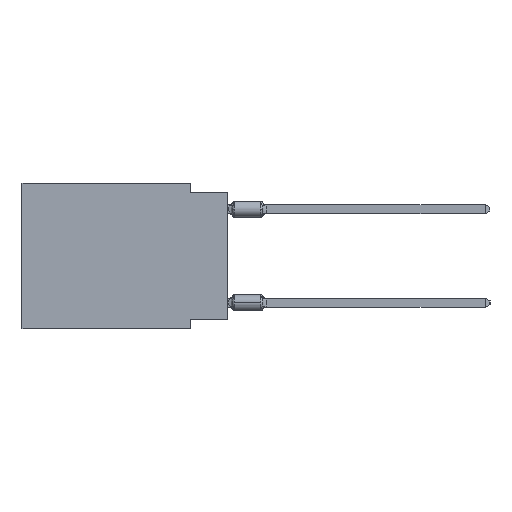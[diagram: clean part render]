
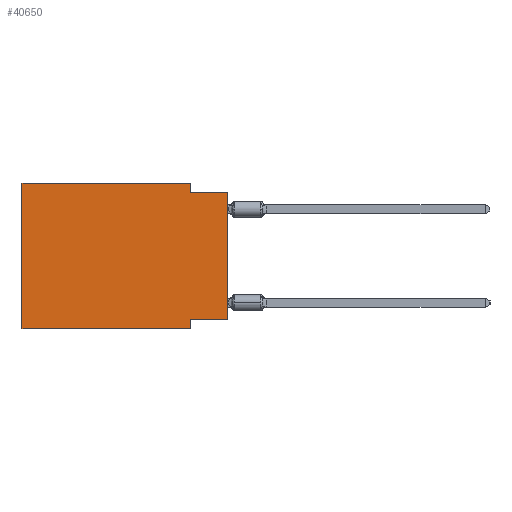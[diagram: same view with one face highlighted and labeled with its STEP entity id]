
A CAD part, left-side view. The second image highlights one B-rep face of the part: STEP entity #40650.
In plain terms, the highlighted planar face has unit normal (-1, 0, 0).
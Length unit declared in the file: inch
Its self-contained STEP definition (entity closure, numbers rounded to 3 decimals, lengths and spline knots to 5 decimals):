
#1346 = VERTEX_POINT ( 'NONE', #27940 ) ;
#1482 = VERTEX_POINT ( 'NONE', #6366 ) ;
#2397 = CARTESIAN_POINT ( 'NONE',  ( 0., 0., -0.025 ) ) ;
#2443 = CARTESIAN_POINT ( 'NONE',  ( 0., 0.1, -0.025 ) ) ;
#3744 = LINE ( 'NONE', #27903, #15398 ) ;
#4629 = FACE_OUTER_BOUND ( 'NONE', #20143, .T. ) ;
#5281 = EDGE_CURVE ( 'NONE', #19329, #8664, #17455, .T. ) ;
#5572 = LINE ( 'NONE', #14890, #19113 ) ;
#6366 = CARTESIAN_POINT ( 'NONE',  ( 0., 0.55, 0. ) ) ;
#7460 = EDGE_CURVE ( 'NONE', #8079, #25161, #27578, .T. ) ;
#7664 = CARTESIAN_POINT ( 'NONE',  ( 0., 0.1, 0. ) ) ;
#8079 = VERTEX_POINT ( 'NONE', #2443 ) ;
#8664 = VERTEX_POINT ( 'NONE', #26353 ) ;
#9581 = CARTESIAN_POINT ( 'NONE',  ( 0., 0., 0. ) ) ;
#10583 = DIRECTION ( 'NONE',  ( 0., 1., 0. ) ) ;
#11356 = EDGE_CURVE ( 'NONE', #19803, #8079, #24972, .T. ) ;
#11784 = VECTOR ( 'NONE', #38459, 39.37008 ) ;
#13032 = ORIENTED_EDGE ( 'NONE', *, *, #17229, .F. ) ;
#13084 = ORIENTED_EDGE ( 'NONE', *, *, #11356, .F. ) ;
#13120 = DIRECTION ( 'NONE',  ( 0., 0., 1. ) ) ;
#14030 = ORIENTED_EDGE ( 'NONE', *, *, #5281, .F. ) ;
#14487 = CARTESIAN_POINT ( 'NONE',  ( 0., 0.55, 0. ) ) ;
#14691 = ORIENTED_EDGE ( 'NONE', *, *, #30767, .T. ) ;
#14890 = CARTESIAN_POINT ( 'NONE',  ( 0., 0.55, 0. ) ) ;
#15280 = EDGE_CURVE ( 'NONE', #20701, #1482, #5572, .T. ) ;
#15398 = VECTOR ( 'NONE', #38090, 39.37008 ) ;
#17229 = EDGE_CURVE ( 'NONE', #1482, #19803, #20938, .T. ) ;
#17455 = LINE ( 'NONE', #24131, #42381 ) ;
#17495 = PLANE ( 'NONE',  #17499 ) ;
#17498 = LINE ( 'NONE', #31476, #43654 ) ;
#17499 = AXIS2_PLACEMENT_3D ( 'NONE', #18152, #21281, #35247 ) ;
#18152 = CARTESIAN_POINT ( 'NONE',  ( 0., 0.55, 0. ) ) ;
#19113 = VECTOR ( 'NONE', #41721, 39.37008 ) ;
#19329 = VERTEX_POINT ( 'NONE', #29270 ) ;
#19803 = VERTEX_POINT ( 'NONE', #32311 ) ;
#20143 = EDGE_LOOP ( 'NONE', ( #14691, #35394, #13084, #13032, #29290, #38434, #33197, #14030 ) ) ;
#20701 = VERTEX_POINT ( 'NONE', #28486 ) ;
#20938 = LINE ( 'NONE', #14487, #11784 ) ;
#21281 = DIRECTION ( 'NONE',  ( 1., 0., 0. ) ) ;
#21282 = DIRECTION ( 'NONE',  ( 0., -1., 0. ) ) ;
#23919 = EDGE_CURVE ( 'NONE', #20701, #1346, #17498, .T. ) ;
#24131 = CARTESIAN_POINT ( 'NONE',  ( 0., 0., -0.365 ) ) ;
#24916 = EDGE_CURVE ( 'NONE', #8664, #1346, #3744, .T. ) ;
#24972 = LINE ( 'NONE', #7664, #25889 ) ;
#25161 = VERTEX_POINT ( 'NONE', #2397 ) ;
#25889 = VECTOR ( 'NONE', #28741, 39.37008 ) ;
#26353 = CARTESIAN_POINT ( 'NONE',  ( 0., 0.1, -0.365 ) ) ;
#27141 = DIRECTION ( 'NONE',  ( 0., -1., 0. ) ) ;
#27578 = LINE ( 'NONE', #40445, #36889 ) ;
#27903 = CARTESIAN_POINT ( 'NONE',  ( 0., 0.1, -0.39 ) ) ;
#27940 = CARTESIAN_POINT ( 'NONE',  ( 0., 0.1, -0.39 ) ) ;
#28486 = CARTESIAN_POINT ( 'NONE',  ( 0., 0.55, -0.39 ) ) ;
#28741 = DIRECTION ( 'NONE',  ( 0., 0., -1. ) ) ;
#29270 = CARTESIAN_POINT ( 'NONE',  ( 0., 0., -0.365 ) ) ;
#29290 = ORIENTED_EDGE ( 'NONE', *, *, #15280, .F. ) ;
#29821 = LINE ( 'NONE', #9581, #33239 ) ;
#30767 = EDGE_CURVE ( 'NONE', #19329, #25161, #29821, .T. ) ;
#31476 = CARTESIAN_POINT ( 'NONE',  ( 0., 0.55, -0.39 ) ) ;
#32311 = CARTESIAN_POINT ( 'NONE',  ( 0., 0.1, 0. ) ) ;
#33197 = ORIENTED_EDGE ( 'NONE', *, *, #24916, .F. ) ;
#33239 = VECTOR ( 'NONE', #13120, 39.37008 ) ;
#35247 = DIRECTION ( 'NONE',  ( 0., 0., -1. ) ) ;
#35394 = ORIENTED_EDGE ( 'NONE', *, *, #7460, .F. ) ;
#36889 = VECTOR ( 'NONE', #27141, 39.37008 ) ;
#38090 = DIRECTION ( 'NONE',  ( 0., 0., -1. ) ) ;
#38434 = ORIENTED_EDGE ( 'NONE', *, *, #23919, .T. ) ;
#38459 = DIRECTION ( 'NONE',  ( 0., -1., 0. ) ) ;
#40445 = CARTESIAN_POINT ( 'NONE',  ( 0., 0., -0.025 ) ) ;
#40650 = ADVANCED_FACE ( 'NONE', ( #4629 ), #17495, .F. ) ;
#41721 = DIRECTION ( 'NONE',  ( 0., 0., 1. ) ) ;
#42381 = VECTOR ( 'NONE', #10583, 39.37008 ) ;
#43654 = VECTOR ( 'NONE', #21282, 39.37008 ) ;
